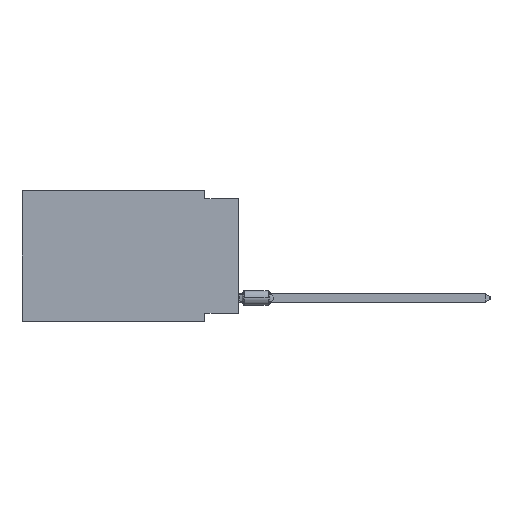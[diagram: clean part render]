
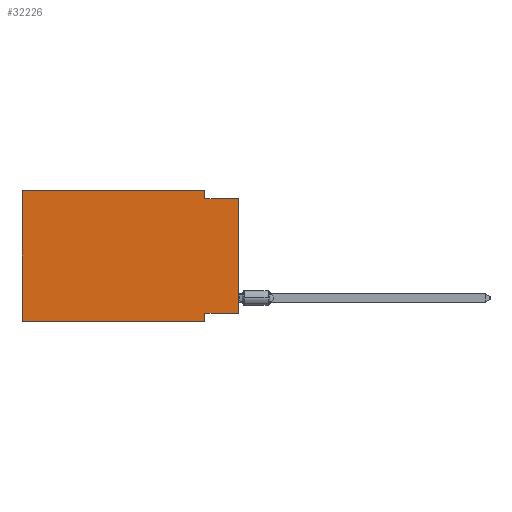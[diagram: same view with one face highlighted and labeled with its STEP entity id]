
A CAD part, left-side view. The second image highlights one B-rep face of the part: STEP entity #32226.
In plain terms, the highlighted planar face has unit normal (-1, 0, 0).
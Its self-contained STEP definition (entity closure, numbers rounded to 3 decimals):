
#1168 = VERTEX_POINT ( 'NONE', #22612 ) ;
#1880 = VERTEX_POINT ( 'NONE', #66834 ) ;
#2072 = VERTEX_POINT ( 'NONE', #21272 ) ;
#2655 = CARTESIAN_POINT ( 'NONE',  ( 0., 0., -9.271 ) ) ;
#2903 = LINE ( 'NONE', #18202, #57440 ) ;
#3328 = ORIENTED_EDGE ( 'NONE', *, *, #69928, .F. ) ;
#5040 = LINE ( 'NONE', #42741, #67159 ) ;
#6803 = EDGE_CURVE ( 'NONE', #43641, #20826, #50320, .T. ) ;
#6810 = ORIENTED_EDGE ( 'NONE', *, *, #67943, .F. ) ;
#7440 = ORIENTED_EDGE ( 'NONE', *, *, #26963, .F. ) ;
#14778 = LINE ( 'NONE', #63154, #47331 ) ;
#15389 = CARTESIAN_POINT ( 'NONE',  ( 0., 2.54, -0.635 ) ) ;
#17265 = CARTESIAN_POINT ( 'NONE',  ( 0., 0., -9.271 ) ) ;
#17401 = VERTEX_POINT ( 'NONE', #15389 ) ;
#18202 = CARTESIAN_POINT ( 'NONE',  ( 0., 0., 0. ) ) ;
#20133 = DIRECTION ( 'NONE',  ( 0., 0., -1. ) ) ;
#20343 = DIRECTION ( 'NONE',  ( 0., -1., 0. ) ) ;
#20826 = VERTEX_POINT ( 'NONE', #66264 ) ;
#21272 = CARTESIAN_POINT ( 'NONE',  ( 0., 2.54, 0. ) ) ;
#22102 = EDGE_CURVE ( 'NONE', #43641, #1168, #2903, .T. ) ;
#22612 = CARTESIAN_POINT ( 'NONE',  ( 0., 0., -0.635 ) ) ;
#23023 = EDGE_LOOP ( 'NONE', ( #31910, #50271, #48347, #7440, #3328, #49745, #6810, #28669 ) ) ;
#24350 = VECTOR ( 'NONE', #60644, 1000. ) ;
#24564 = VECTOR ( 'NONE', #58799, 1000. ) ;
#25127 = FACE_OUTER_BOUND ( 'NONE', #23023, .T. ) ;
#25191 = VERTEX_POINT ( 'NONE', #66934 ) ;
#26963 = EDGE_CURVE ( 'NONE', #32093, #2072, #5040, .T. ) ;
#28669 = ORIENTED_EDGE ( 'NONE', *, *, #6803, .F. ) ;
#31804 = LINE ( 'NONE', #64147, #24564 ) ;
#31910 = ORIENTED_EDGE ( 'NONE', *, *, #22102, .T. ) ;
#32093 = VERTEX_POINT ( 'NONE', #40080 ) ;
#32226 = ADVANCED_FACE ( 'NONE', ( #25127 ), #47502, .F. ) ;
#32986 = CARTESIAN_POINT ( 'NONE',  ( 0., 16.383, -9.906 ) ) ;
#34049 = CARTESIAN_POINT ( 'NONE',  ( 0., 0., -0.635 ) ) ;
#34173 = LINE ( 'NONE', #62583, #64255 ) ;
#36141 = DIRECTION ( 'NONE',  ( 0., 0., 1. ) ) ;
#40080 = CARTESIAN_POINT ( 'NONE',  ( 0., 16.383, 0. ) ) ;
#40419 = LINE ( 'NONE', #34049, #63109 ) ;
#42741 = CARTESIAN_POINT ( 'NONE',  ( 0., 16.383, 0. ) ) ;
#43641 = VERTEX_POINT ( 'NONE', #2655 ) ;
#45527 = DIRECTION ( 'NONE',  ( 0., 0., -1. ) ) ;
#45960 = EDGE_CURVE ( 'NONE', #2072, #17401, #34173, .T. ) ;
#46281 = DIRECTION ( 'NONE',  ( 0., 0., 1. ) ) ;
#47331 = VECTOR ( 'NONE', #36141, 1000. ) ;
#47502 = PLANE ( 'NONE',  #69787 ) ;
#47843 = CARTESIAN_POINT ( 'NONE',  ( 0., 16.383, 0. ) ) ;
#48347 = ORIENTED_EDGE ( 'NONE', *, *, #45960, .F. ) ;
#49332 = LINE ( 'NONE', #32986, #61982 ) ;
#49745 = ORIENTED_EDGE ( 'NONE', *, *, #53509, .T. ) ;
#50271 = ORIENTED_EDGE ( 'NONE', *, *, #53608, .F. ) ;
#50320 = LINE ( 'NONE', #17265, #24350 ) ;
#53509 = EDGE_CURVE ( 'NONE', #1880, #25191, #49332, .T. ) ;
#53608 = EDGE_CURVE ( 'NONE', #17401, #1168, #40419, .T. ) ;
#57440 = VECTOR ( 'NONE', #46281, 1000. ) ;
#58799 = DIRECTION ( 'NONE',  ( 0., 0., -1. ) ) ;
#60644 = DIRECTION ( 'NONE',  ( 0., 1., 0. ) ) ;
#61062 = DIRECTION ( 'NONE',  ( 0., -1., 0. ) ) ;
#61982 = VECTOR ( 'NONE', #65329, 1000. ) ;
#62583 = CARTESIAN_POINT ( 'NONE',  ( 0., 2.54, 0. ) ) ;
#62812 = DIRECTION ( 'NONE',  ( 1., 0., 0. ) ) ;
#63109 = VECTOR ( 'NONE', #61062, 1000. ) ;
#63154 = CARTESIAN_POINT ( 'NONE',  ( 0., 16.383, 0. ) ) ;
#64147 = CARTESIAN_POINT ( 'NONE',  ( 0., 2.54, -9.906 ) ) ;
#64255 = VECTOR ( 'NONE', #45527, 1000. ) ;
#65329 = DIRECTION ( 'NONE',  ( 0., -1., 0. ) ) ;
#66264 = CARTESIAN_POINT ( 'NONE',  ( 0., 2.54, -9.271 ) ) ;
#66834 = CARTESIAN_POINT ( 'NONE',  ( 0., 16.383, -9.906 ) ) ;
#66934 = CARTESIAN_POINT ( 'NONE',  ( 0., 2.54, -9.906 ) ) ;
#67159 = VECTOR ( 'NONE', #20343, 1000. ) ;
#67943 = EDGE_CURVE ( 'NONE', #20826, #25191, #31804, .T. ) ;
#69787 = AXIS2_PLACEMENT_3D ( 'NONE', #47843, #62812, #20133 ) ;
#69928 = EDGE_CURVE ( 'NONE', #1880, #32093, #14778, .T. ) ;
